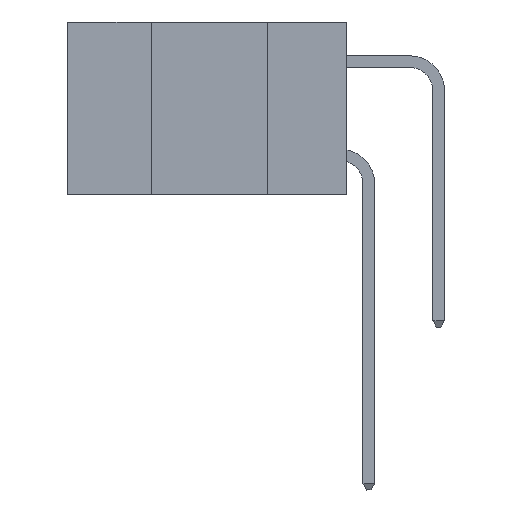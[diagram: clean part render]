
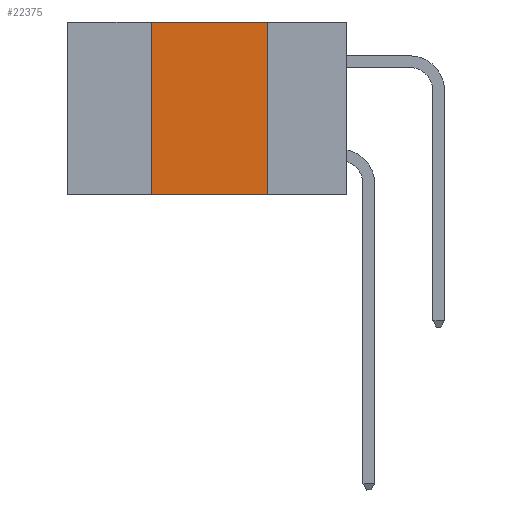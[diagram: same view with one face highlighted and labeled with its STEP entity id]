
A CAD part, left-side view. The second image highlights one B-rep face of the part: STEP entity #22375.
In plain terms, the highlighted planar face has unit normal (-1, 0, 0).
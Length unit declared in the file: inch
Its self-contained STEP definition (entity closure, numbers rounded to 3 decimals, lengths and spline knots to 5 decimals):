
#330 = ORIENTED_EDGE ( 'NONE', *, *, #12734, .F. ) ;
#2064 = CARTESIAN_POINT ( 'NONE',  ( 0., 0.17, 0. ) ) ;
#2286 = CARTESIAN_POINT ( 'NONE',  ( 0., 0.42, -0.37 ) ) ;
#3663 = EDGE_LOOP ( 'NONE', ( #16086, #7703, #330, #27393 ) ) ;
#5860 = VERTEX_POINT ( 'NONE', #2286 ) ;
#7703 = ORIENTED_EDGE ( 'NONE', *, *, #29150, .F. ) ;
#10329 = VERTEX_POINT ( 'NONE', #2064 ) ;
#10540 = AXIS2_PLACEMENT_3D ( 'NONE', #28953, #14474, #29282 ) ;
#10937 = VECTOR ( 'NONE', #20688, 39.37008 ) ;
#11329 = LINE ( 'NONE', #23577, #10937 ) ;
#11870 = PLANE ( 'NONE',  #10540 ) ;
#12075 = CARTESIAN_POINT ( 'NONE',  ( 0., 0.42, 0. ) ) ;
#12319 = VECTOR ( 'NONE', #29787, 39.37008 ) ;
#12697 = CARTESIAN_POINT ( 'NONE',  ( 0., 0.6, 0. ) ) ;
#12734 = EDGE_CURVE ( 'NONE', #5860, #29898, #28671, .T. ) ;
#14474 = DIRECTION ( 'NONE',  ( 1., 0., 0. ) ) ;
#14793 = VECTOR ( 'NONE', #30327, 39.37008 ) ;
#15411 = EDGE_CURVE ( 'NONE', #10329, #24689, #22739, .T. ) ;
#16086 = ORIENTED_EDGE ( 'NONE', *, *, #15411, .F. ) ;
#16997 = VECTOR ( 'NONE', #17088, 39.37008 ) ;
#17088 = DIRECTION ( 'NONE',  ( 0., 0., 1. ) ) ;
#19954 = LINE ( 'NONE', #12697, #12319 ) ;
#20087 = EDGE_CURVE ( 'NONE', #5860, #24689, #11329, .T. ) ;
#20688 = DIRECTION ( 'NONE',  ( 0., -1., 0. ) ) ;
#22187 = FACE_OUTER_BOUND ( 'NONE', #3663, .T. ) ;
#22375 = ADVANCED_FACE ( 'NONE', ( #22187 ), #11870, .F. ) ;
#22739 = LINE ( 'NONE', #30006, #14793 ) ;
#23577 = CARTESIAN_POINT ( 'NONE',  ( 0., 0.6, -0.37 ) ) ;
#24689 = VERTEX_POINT ( 'NONE', #26374 ) ;
#26161 = CARTESIAN_POINT ( 'NONE',  ( 0., 0.42, 0. ) ) ;
#26374 = CARTESIAN_POINT ( 'NONE',  ( 0., 0.17, -0.37 ) ) ;
#27393 = ORIENTED_EDGE ( 'NONE', *, *, #20087, .T. ) ;
#28671 = LINE ( 'NONE', #12075, #16997 ) ;
#28953 = CARTESIAN_POINT ( 'NONE',  ( 0., 0.6, 0. ) ) ;
#29150 = EDGE_CURVE ( 'NONE', #29898, #10329, #19954, .T. ) ;
#29282 = DIRECTION ( 'NONE',  ( 0., 0., -1. ) ) ;
#29787 = DIRECTION ( 'NONE',  ( 0., -1., 0. ) ) ;
#29898 = VERTEX_POINT ( 'NONE', #26161 ) ;
#30006 = CARTESIAN_POINT ( 'NONE',  ( 0., 0.17, 0. ) ) ;
#30327 = DIRECTION ( 'NONE',  ( 0., 0., -1. ) ) ;
